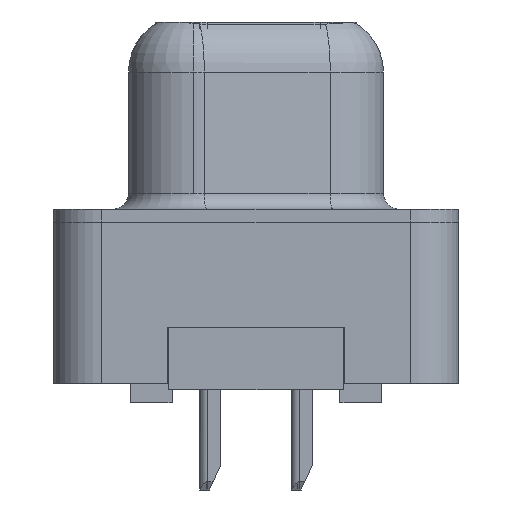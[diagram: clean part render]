
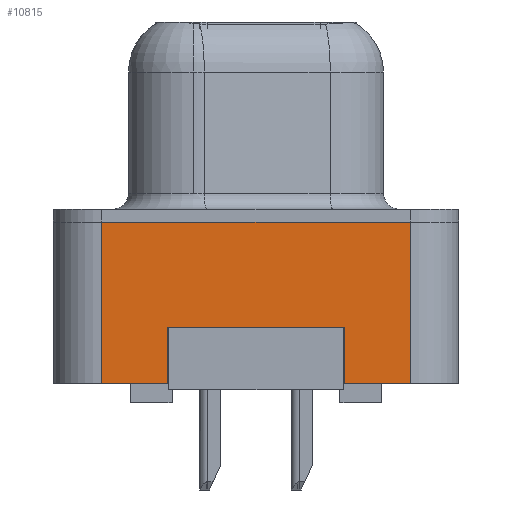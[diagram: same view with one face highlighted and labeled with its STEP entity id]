
A CAD part, left-side view. The second image highlights one B-rep face of the part: STEP entity #10815.
In plain terms, the highlighted planar face has unit normal (-1, 0, 0).
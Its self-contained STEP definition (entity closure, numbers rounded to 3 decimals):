
#160 = VECTOR ( 'NONE', #2774, 1000. ) ;
#217 = CARTESIAN_POINT ( 'NONE',  ( -2.995, 2.75, -3.25 ) ) ;
#451 = LINE ( 'NONE', #3576, #15675 ) ;
#2122 = VERTEX_POINT ( 'NONE', #7135 ) ;
#2293 = CARTESIAN_POINT ( 'NONE',  ( -2.995, 2.75, -3.25 ) ) ;
#2384 = VECTOR ( 'NONE', #12373, 1000. ) ;
#2774 = DIRECTION ( 'NONE',  ( 0., 0., -1. ) ) ;
#3240 = ORIENTED_EDGE ( 'NONE', *, *, #19117, .F. ) ;
#3320 = DIRECTION ( 'NONE',  ( 0., 1., 0. ) ) ;
#3341 = DIRECTION ( 'NONE',  ( 0., 0., -1. ) ) ;
#3576 = CARTESIAN_POINT ( 'NONE',  ( -2.995, 4.775, -5. ) ) ;
#3809 = CARTESIAN_POINT ( 'NONE',  ( -2.995, -4.775, 0. ) ) ;
#4375 = CARTESIAN_POINT ( 'NONE',  ( -2.995, -4.775, -5. ) ) ;
#5332 = VECTOR ( 'NONE', #3341, 1000. ) ;
#5346 = DIRECTION ( 'NONE',  ( 0., 0., 1. ) ) ;
#5919 = EDGE_LOOP ( 'NONE', ( #8940, #7754, #7251, #13383, #12056, #8366, #3240, #11680 ) ) ;
#6374 = LINE ( 'NONE', #217, #5332 ) ;
#6429 = AXIS2_PLACEMENT_3D ( 'NONE', #14826, #16296, #5346 ) ;
#6558 = VERTEX_POINT ( 'NONE', #3809 ) ;
#6874 = CARTESIAN_POINT ( 'NONE',  ( -2.995, -4.775, -5. ) ) ;
#7135 = CARTESIAN_POINT ( 'NONE',  ( -2.995, 4.775, -5. ) ) ;
#7251 = ORIENTED_EDGE ( 'NONE', *, *, #8273, .T. ) ;
#7260 = CARTESIAN_POINT ( 'NONE',  ( -2.995, -2.75, -3.25 ) ) ;
#7754 = ORIENTED_EDGE ( 'NONE', *, *, #16897, .T. ) ;
#8273 = EDGE_CURVE ( 'NONE', #17073, #6558, #15212, .T. ) ;
#8365 = VECTOR ( 'NONE', #15107, 1000. ) ;
#8366 = ORIENTED_EDGE ( 'NONE', *, *, #13481, .T. ) ;
#8406 = EDGE_CURVE ( 'NONE', #15931, #6558, #13638, .T. ) ;
#8746 = LINE ( 'NONE', #10412, #16182 ) ;
#8940 = ORIENTED_EDGE ( 'NONE', *, *, #12171, .T. ) ;
#9860 = LINE ( 'NONE', #17613, #11183 ) ;
#10131 = DIRECTION ( 'NONE',  ( 0., 0., 1. ) ) ;
#10401 = CARTESIAN_POINT ( 'NONE',  ( -2.995, -4.775, -5. ) ) ;
#10412 = CARTESIAN_POINT ( 'NONE',  ( -2.995, -4.775, -5. ) ) ;
#10815 = ADVANCED_FACE ( 'NONE', ( #11477 ), #16397, .T. ) ;
#11183 = VECTOR ( 'NONE', #3320, 1000. ) ;
#11477 = FACE_OUTER_BOUND ( 'NONE', #5919, .T. ) ;
#11680 = ORIENTED_EDGE ( 'NONE', *, *, #15284, .F. ) ;
#12056 = ORIENTED_EDGE ( 'NONE', *, *, #20154, .F. ) ;
#12171 = EDGE_CURVE ( 'NONE', #15310, #12589, #18227, .T. ) ;
#12373 = DIRECTION ( 'NONE',  ( 0., -1., 0. ) ) ;
#12589 = VERTEX_POINT ( 'NONE', #15067 ) ;
#13383 = ORIENTED_EDGE ( 'NONE', *, *, #8406, .F. ) ;
#13481 = EDGE_CURVE ( 'NONE', #2122, #19832, #8746, .T. ) ;
#13638 = LINE ( 'NONE', #20015, #2384 ) ;
#13695 = CARTESIAN_POINT ( 'NONE',  ( -2.995, 2.75, -5. ) ) ;
#14826 = CARTESIAN_POINT ( 'NONE',  ( -2.995, -4.775, -5. ) ) ;
#15067 = CARTESIAN_POINT ( 'NONE',  ( -2.995, -2.75, -5. ) ) ;
#15107 = DIRECTION ( 'NONE',  ( 0., 0., 1. ) ) ;
#15212 = LINE ( 'NONE', #10401, #8365 ) ;
#15284 = EDGE_CURVE ( 'NONE', #15310, #20540, #9860, .T. ) ;
#15310 = VERTEX_POINT ( 'NONE', #18440 ) ;
#15568 = VECTOR ( 'NONE', #18140, 1000. ) ;
#15675 = VECTOR ( 'NONE', #10131, 1000. ) ;
#15931 = VERTEX_POINT ( 'NONE', #19215 ) ;
#16182 = VECTOR ( 'NONE', #18257, 1000. ) ;
#16296 = DIRECTION ( 'NONE',  ( -1., 0., 0. ) ) ;
#16397 = PLANE ( 'NONE',  #6429 ) ;
#16587 = LINE ( 'NONE', #6874, #15568 ) ;
#16897 = EDGE_CURVE ( 'NONE', #12589, #17073, #16587, .T. ) ;
#17073 = VERTEX_POINT ( 'NONE', #4375 ) ;
#17613 = CARTESIAN_POINT ( 'NONE',  ( -2.995, 2.75, -3.25 ) ) ;
#18140 = DIRECTION ( 'NONE',  ( 0., -1., 0. ) ) ;
#18227 = LINE ( 'NONE', #7260, #160 ) ;
#18257 = DIRECTION ( 'NONE',  ( 0., -1., 0. ) ) ;
#18440 = CARTESIAN_POINT ( 'NONE',  ( -2.995, -2.75, -3.25 ) ) ;
#19117 = EDGE_CURVE ( 'NONE', #20540, #19832, #6374, .T. ) ;
#19215 = CARTESIAN_POINT ( 'NONE',  ( -2.995, 4.775, 0. ) ) ;
#19832 = VERTEX_POINT ( 'NONE', #13695 ) ;
#20015 = CARTESIAN_POINT ( 'NONE',  ( -2.995, -4.775, 0. ) ) ;
#20154 = EDGE_CURVE ( 'NONE', #2122, #15931, #451, .T. ) ;
#20540 = VERTEX_POINT ( 'NONE', #2293 ) ;
